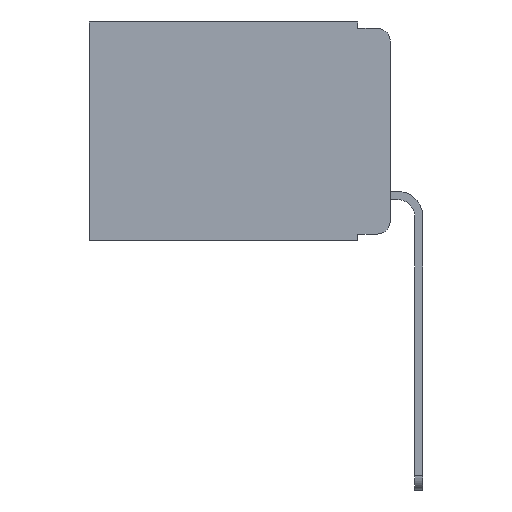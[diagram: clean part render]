
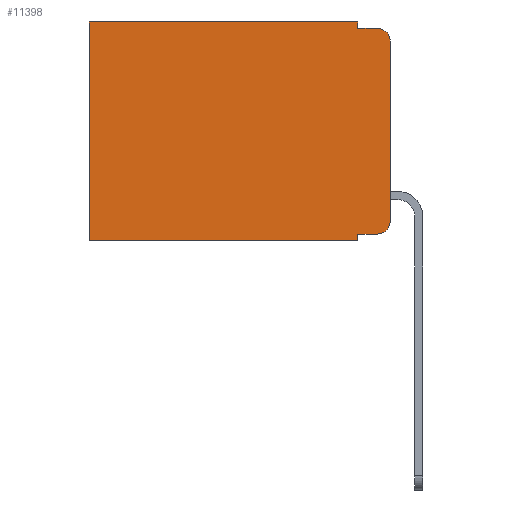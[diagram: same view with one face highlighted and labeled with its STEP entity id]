
A CAD part, left-side view. The second image highlights one B-rep face of the part: STEP entity #11398.
In plain terms, the highlighted planar face has unit normal (-1, 0, 0).
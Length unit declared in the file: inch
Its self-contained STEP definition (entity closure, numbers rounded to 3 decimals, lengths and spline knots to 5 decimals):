
#143 = LINE ( 'NONE', #7254, #11328 ) ;
#247 = EDGE_CURVE ( 'NONE', #4044, #11834, #3564, .T. ) ;
#271 = EDGE_CURVE ( 'NONE', #9848, #9665, #8147, .T. ) ;
#363 = EDGE_CURVE ( 'NONE', #1457, #8541, #6446, .T. ) ;
#388 = ORIENTED_EDGE ( 'NONE', *, *, #247, .F. ) ;
#418 = AXIS2_PLACEMENT_3D ( 'NONE', #10440, #521, #11387 ) ;
#427 = EDGE_CURVE ( 'NONE', #1457, #883, #5616, .T. ) ;
#493 = FACE_OUTER_BOUND ( 'NONE', #5617, .T. ) ;
#521 = DIRECTION ( 'NONE',  ( -1., 0., 0. ) ) ;
#545 = VECTOR ( 'NONE', #2870, 39.37008 ) ;
#624 = CARTESIAN_POINT ( 'NONE',  ( 0.298, 0., 0. ) ) ;
#883 = VERTEX_POINT ( 'NONE', #11155 ) ;
#898 = CARTESIAN_POINT ( 'NONE',  ( 0.298, 0.02, -0.01 ) ) ;
#992 = VERTEX_POINT ( 'NONE', #11516 ) ;
#1005 = DIRECTION ( 'NONE',  ( 0., 1., 0. ) ) ;
#1457 = VERTEX_POINT ( 'NONE', #5795 ) ;
#1519 = CARTESIAN_POINT ( 'NONE',  ( 0.298, 0.473, 0. ) ) ;
#1623 = DIRECTION ( 'NONE',  ( 0., 0., -1. ) ) ;
#1890 = AXIS2_PLACEMENT_3D ( 'NONE', #8688, #8734, #5290 ) ;
#2068 = CIRCLE ( 'NONE', #418, 0.02 ) ;
#2130 = EDGE_CURVE ( 'NONE', #4044, #9848, #12020, .T. ) ;
#2332 = EDGE_CURVE ( 'NONE', #11834, #7166, #3335, .T. ) ;
#2870 = DIRECTION ( 'NONE',  ( 0., -1., 0. ) ) ;
#2976 = EDGE_CURVE ( 'NONE', #992, #7166, #2068, .T. ) ;
#3001 = EDGE_CURVE ( 'NONE', #883, #10685, #10933, .T. ) ;
#3104 = VECTOR ( 'NONE', #10419, 39.37008 ) ;
#3324 = EDGE_CURVE ( 'NONE', #8541, #9665, #143, .T. ) ;
#3335 = LINE ( 'NONE', #4968, #545 ) ;
#3564 = LINE ( 'NONE', #6312, #4163 ) ;
#3715 = VECTOR ( 'NONE', #9649, 39.37008 ) ;
#3732 = CARTESIAN_POINT ( 'NONE',  ( 0.298, 0.051, 0. ) ) ;
#4044 = VERTEX_POINT ( 'NONE', #11084 ) ;
#4112 = ORIENTED_EDGE ( 'NONE', *, *, #363, .F. ) ;
#4163 = VECTOR ( 'NONE', #5859, 39.37008 ) ;
#4343 = EDGE_CURVE ( 'NONE', #992, #10685, #6469, .T. ) ;
#4432 = CARTESIAN_POINT ( 'NONE',  ( 0.298, 0., 0. ) ) ;
#4554 = AXIS2_PLACEMENT_3D ( 'NONE', #4432, #5385, #11547 ) ;
#4947 = VECTOR ( 'NONE', #1005, 39.37008 ) ;
#4968 = CARTESIAN_POINT ( 'NONE',  ( 0.298, 0.051, -0.01 ) ) ;
#5121 = ORIENTED_EDGE ( 'NONE', *, *, #2976, .T. ) ;
#5125 = CARTESIAN_POINT ( 'NONE',  ( 0.298, 0.051, -0.01 ) ) ;
#5290 = DIRECTION ( 'NONE',  ( 0., 0., -1. ) ) ;
#5385 = DIRECTION ( 'NONE',  ( 1., 0., 0. ) ) ;
#5410 = DIRECTION ( 'NONE',  ( 0., 1., 0. ) ) ;
#5616 = LINE ( 'NONE', #9920, #3104 ) ;
#5617 = EDGE_LOOP ( 'NONE', ( #9331, #5121, #9885, #388, #8096, #8374, #6270, #4112, #6831, #7118 ) ) ;
#5795 = CARTESIAN_POINT ( 'NONE',  ( 0.298, 0.051, -0.333 ) ) ;
#5810 = CARTESIAN_POINT ( 'NONE',  ( 0.298, 0.473, 0. ) ) ;
#5859 = DIRECTION ( 'NONE',  ( 0., 0., -1. ) ) ;
#6026 = DIRECTION ( 'NONE',  ( 0., 0., -1. ) ) ;
#6270 = ORIENTED_EDGE ( 'NONE', *, *, #3324, .F. ) ;
#6312 = CARTESIAN_POINT ( 'NONE',  ( 0.298, 0.051, 0. ) ) ;
#6446 = LINE ( 'NONE', #3732, #3715 ) ;
#6469 = LINE ( 'NONE', #11983, #11432 ) ;
#6831 = ORIENTED_EDGE ( 'NONE', *, *, #427, .T. ) ;
#7118 = ORIENTED_EDGE ( 'NONE', *, *, #3001, .T. ) ;
#7166 = VERTEX_POINT ( 'NONE', #898 ) ;
#7254 = CARTESIAN_POINT ( 'NONE',  ( 0.298, 0., -0.343 ) ) ;
#7304 = CARTESIAN_POINT ( 'NONE',  ( 0.298, 0.473, -0.343 ) ) ;
#7424 = CARTESIAN_POINT ( 'NONE',  ( 0.298, 0.051, -0.343 ) ) ;
#7872 = VECTOR ( 'NONE', #6026, 39.37008 ) ;
#8096 = ORIENTED_EDGE ( 'NONE', *, *, #2130, .T. ) ;
#8147 = LINE ( 'NONE', #1519, #7872 ) ;
#8374 = ORIENTED_EDGE ( 'NONE', *, *, #271, .T. ) ;
#8541 = VERTEX_POINT ( 'NONE', #7424 ) ;
#8688 = CARTESIAN_POINT ( 'NONE',  ( 0.298, 0.02, -0.313 ) ) ;
#8734 = DIRECTION ( 'NONE',  ( -1., 0., 0. ) ) ;
#9331 = ORIENTED_EDGE ( 'NONE', *, *, #4343, .F. ) ;
#9649 = DIRECTION ( 'NONE',  ( 0., 0., -1. ) ) ;
#9665 = VERTEX_POINT ( 'NONE', #7304 ) ;
#9826 = PLANE ( 'NONE',  #4554 ) ;
#9848 = VERTEX_POINT ( 'NONE', #5810 ) ;
#9885 = ORIENTED_EDGE ( 'NONE', *, *, #2332, .F. ) ;
#9920 = CARTESIAN_POINT ( 'NONE',  ( 0.298, 0.051, -0.333 ) ) ;
#10419 = DIRECTION ( 'NONE',  ( 0., -1., 0. ) ) ;
#10440 = CARTESIAN_POINT ( 'NONE',  ( 0.298, 0.02, -0.03 ) ) ;
#10649 = CARTESIAN_POINT ( 'NONE',  ( 0.298, 0., -0.313 ) ) ;
#10685 = VERTEX_POINT ( 'NONE', #10649 ) ;
#10933 = CIRCLE ( 'NONE', #1890, 0.02 ) ;
#11084 = CARTESIAN_POINT ( 'NONE',  ( 0.298, 0.051, 0. ) ) ;
#11155 = CARTESIAN_POINT ( 'NONE',  ( 0.298, 0.02, -0.333 ) ) ;
#11328 = VECTOR ( 'NONE', #5410, 39.37008 ) ;
#11387 = DIRECTION ( 'NONE',  ( 0., 0., -1. ) ) ;
#11398 = ADVANCED_FACE ( 'NONE', ( #493 ), #9826, .F. ) ;
#11432 = VECTOR ( 'NONE', #1623, 39.37008 ) ;
#11516 = CARTESIAN_POINT ( 'NONE',  ( 0.298, 0., -0.03 ) ) ;
#11547 = DIRECTION ( 'NONE',  ( 0., 0., -1. ) ) ;
#11834 = VERTEX_POINT ( 'NONE', #5125 ) ;
#11983 = CARTESIAN_POINT ( 'NONE',  ( 0.298, 0., 0. ) ) ;
#12020 = LINE ( 'NONE', #624, #4947 ) ;
